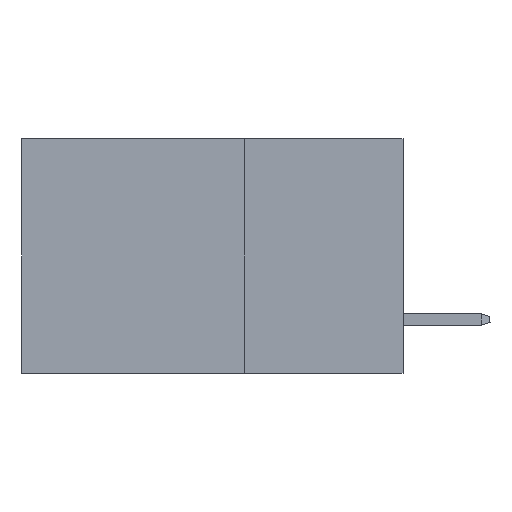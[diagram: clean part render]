
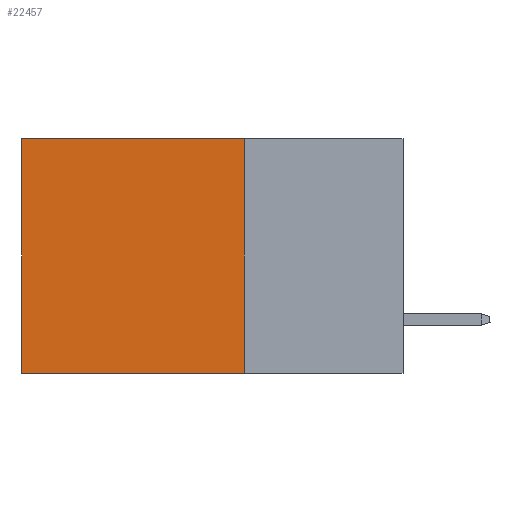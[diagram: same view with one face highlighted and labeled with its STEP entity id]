
A CAD part, left-side view. The second image highlights one B-rep face of the part: STEP entity #22457.
In plain terms, the highlighted planar face has unit normal (-1, 0, 0).
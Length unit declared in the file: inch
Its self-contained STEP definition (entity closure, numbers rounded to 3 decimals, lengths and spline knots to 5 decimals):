
#2743 = LINE ( 'NONE', #12496, #15423 ) ;
#3204 = VERTEX_POINT ( 'NONE', #27099 ) ;
#3719 = LINE ( 'NONE', #17977, #23452 ) ;
#5147 = VERTEX_POINT ( 'NONE', #10452 ) ;
#5366 = VERTEX_POINT ( 'NONE', #9821 ) ;
#5775 = DIRECTION ( 'NONE',  ( 1., 0., 0. ) ) ;
#6188 = CARTESIAN_POINT ( 'NONE',  ( 0.2875, 0.25, 0. ) ) ;
#6325 = AXIS2_PLACEMENT_3D ( 'NONE', #6188, #5775, #14646 ) ;
#6622 = EDGE_CURVE ( 'NONE', #3204, #27180, #21816, .T. ) ;
#7265 = DIRECTION ( 'NONE',  ( 0., 0., -1. ) ) ;
#7402 = EDGE_CURVE ( 'NONE', #5366, #3204, #2743, .T. ) ;
#7879 = VECTOR ( 'NONE', #7265, 39.37008 ) ;
#8295 = FACE_OUTER_BOUND ( 'NONE', #20643, .T. ) ;
#9561 = ORIENTED_EDGE ( 'NONE', *, *, #19441, .F. ) ;
#9821 = CARTESIAN_POINT ( 'NONE',  ( 0.2875, 0.25, 0. ) ) ;
#10452 = CARTESIAN_POINT ( 'NONE',  ( 0.2875, 0.25, -0.37 ) ) ;
#10548 = DIRECTION ( 'NONE',  ( 0., 1., 0. ) ) ;
#11458 = EDGE_CURVE ( 'NONE', #5147, #27180, #26275, .T. ) ;
#12168 = PLANE ( 'NONE',  #6325 ) ;
#12496 = CARTESIAN_POINT ( 'NONE',  ( 0.2875, 0.25, 0. ) ) ;
#14646 = DIRECTION ( 'NONE',  ( 0., 0., -1. ) ) ;
#15401 = CARTESIAN_POINT ( 'NONE',  ( 0.2875, 0.6, -0.37 ) ) ;
#15423 = VECTOR ( 'NONE', #10548, 39.37008 ) ;
#17977 = CARTESIAN_POINT ( 'NONE',  ( 0.2875, 0.25, 0. ) ) ;
#18110 = DIRECTION ( 'NONE',  ( 0., 0., -1. ) ) ;
#19441 = EDGE_CURVE ( 'NONE', #5366, #5147, #3719, .T. ) ;
#20643 = EDGE_LOOP ( 'NONE', ( #21589, #21675, #9561, #20670 ) ) ;
#20670 = ORIENTED_EDGE ( 'NONE', *, *, #7402, .T. ) ;
#21589 = ORIENTED_EDGE ( 'NONE', *, *, #6622, .T. ) ;
#21675 = ORIENTED_EDGE ( 'NONE', *, *, #11458, .F. ) ;
#21816 = LINE ( 'NONE', #25931, #7879 ) ;
#22025 = DIRECTION ( 'NONE',  ( 0., 1., 0. ) ) ;
#22457 = ADVANCED_FACE ( 'NONE', ( #8295 ), #12168, .F. ) ;
#23452 = VECTOR ( 'NONE', #18110, 39.37008 ) ;
#25658 = VECTOR ( 'NONE', #22025, 39.37008 ) ;
#25931 = CARTESIAN_POINT ( 'NONE',  ( 0.2875, 0.6, 0. ) ) ;
#26004 = CARTESIAN_POINT ( 'NONE',  ( 0.2875, 0.25, -0.37 ) ) ;
#26275 = LINE ( 'NONE', #26004, #25658 ) ;
#27099 = CARTESIAN_POINT ( 'NONE',  ( 0.2875, 0.6, 0. ) ) ;
#27180 = VERTEX_POINT ( 'NONE', #15401 ) ;
